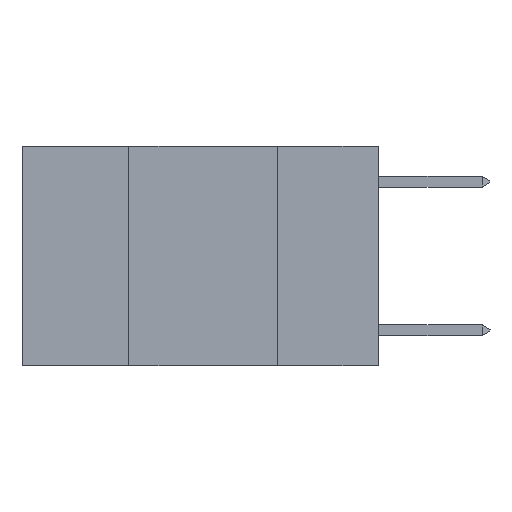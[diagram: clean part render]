
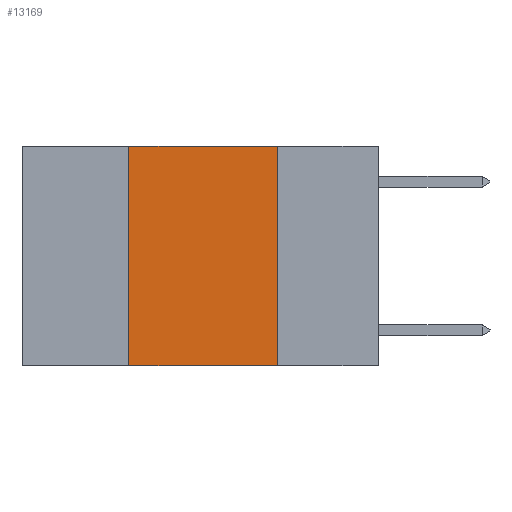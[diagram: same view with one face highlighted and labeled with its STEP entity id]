
A CAD part, left-side view. The second image highlights one B-rep face of the part: STEP entity #13169.
In plain terms, the highlighted planar face has unit normal (-1, 0, 0).
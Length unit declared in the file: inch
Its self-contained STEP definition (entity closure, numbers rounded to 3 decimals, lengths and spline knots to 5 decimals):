
#626 = VECTOR ( 'NONE', #14587, 39.37008 ) ;
#720 = DIRECTION ( 'NONE',  ( 0., -1., 0. ) ) ;
#1171 = CARTESIAN_POINT ( 'NONE',  ( 0., 0.17, 0. ) ) ;
#1371 = CARTESIAN_POINT ( 'NONE',  ( 0., 0.42, 0. ) ) ;
#1835 = CARTESIAN_POINT ( 'NONE',  ( 0., 0.17, -0.37 ) ) ;
#2022 = VECTOR ( 'NONE', #11885, 39.37008 ) ;
#2030 = CARTESIAN_POINT ( 'NONE',  ( 0., 0.42, 0. ) ) ;
#2134 = AXIS2_PLACEMENT_3D ( 'NONE', #11054, #3681, #12270 ) ;
#2771 = VERTEX_POINT ( 'NONE', #14185 ) ;
#2865 = EDGE_CURVE ( 'NONE', #2771, #3199, #5720, .T. ) ;
#3199 = VERTEX_POINT ( 'NONE', #1371 ) ;
#3681 = DIRECTION ( 'NONE',  ( 1., 0., 0. ) ) ;
#3682 = FACE_OUTER_BOUND ( 'NONE', #3722, .T. ) ;
#3722 = EDGE_LOOP ( 'NONE', ( #11444, #6055, #15083, #15769 ) ) ;
#4634 = LINE ( 'NONE', #1171, #11165 ) ;
#5645 = CARTESIAN_POINT ( 'NONE',  ( 0., 0.6, 0. ) ) ;
#5720 = LINE ( 'NONE', #2030, #2022 ) ;
#6055 = ORIENTED_EDGE ( 'NONE', *, *, #12918, .F. ) ;
#7186 = VECTOR ( 'NONE', #720, 39.37008 ) ;
#8495 = CARTESIAN_POINT ( 'NONE',  ( 0., 0.6, -0.37 ) ) ;
#8538 = PLANE ( 'NONE',  #2134 ) ;
#8570 = DIRECTION ( 'NONE',  ( 0., 0., -1. ) ) ;
#8956 = CARTESIAN_POINT ( 'NONE',  ( 0., 0.17, 0. ) ) ;
#10068 = LINE ( 'NONE', #8495, #626 ) ;
#10447 = LINE ( 'NONE', #5645, #7186 ) ;
#11054 = CARTESIAN_POINT ( 'NONE',  ( 0., 0.6, 0. ) ) ;
#11165 = VECTOR ( 'NONE', #8570, 39.37008 ) ;
#11444 = ORIENTED_EDGE ( 'NONE', *, *, #13781, .F. ) ;
#11885 = DIRECTION ( 'NONE',  ( 0., 0., 1. ) ) ;
#12048 = VERTEX_POINT ( 'NONE', #8956 ) ;
#12270 = DIRECTION ( 'NONE',  ( 0., 0., -1. ) ) ;
#12456 = EDGE_CURVE ( 'NONE', #2771, #14823, #10068, .T. ) ;
#12918 = EDGE_CURVE ( 'NONE', #3199, #12048, #10447, .T. ) ;
#13169 = ADVANCED_FACE ( 'NONE', ( #3682 ), #8538, .F. ) ;
#13781 = EDGE_CURVE ( 'NONE', #12048, #14823, #4634, .T. ) ;
#14185 = CARTESIAN_POINT ( 'NONE',  ( 0., 0.42, -0.37 ) ) ;
#14587 = DIRECTION ( 'NONE',  ( 0., -1., 0. ) ) ;
#14823 = VERTEX_POINT ( 'NONE', #1835 ) ;
#15083 = ORIENTED_EDGE ( 'NONE', *, *, #2865, .F. ) ;
#15769 = ORIENTED_EDGE ( 'NONE', *, *, #12456, .T. ) ;
